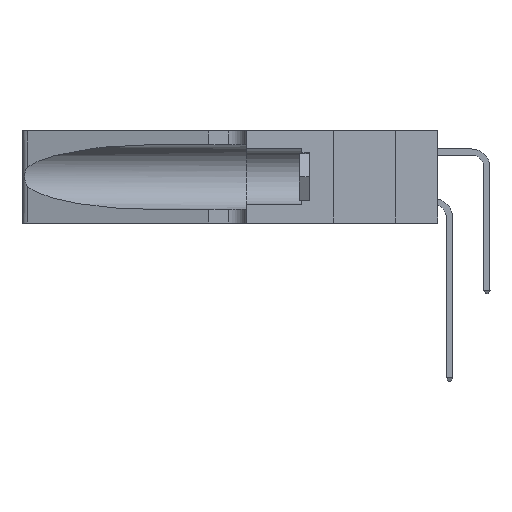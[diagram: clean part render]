
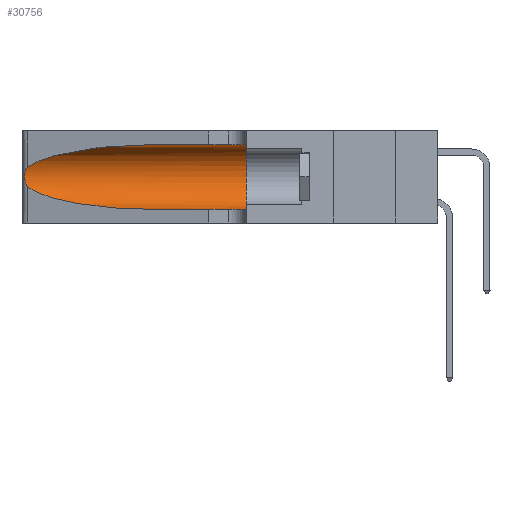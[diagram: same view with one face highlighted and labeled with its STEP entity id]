
A CAD part, left-side view. The second image highlights one B-rep face of the part: STEP entity #30756.
In plain terms, the highlighted cylindrical face has radius 3.308 mm (diameter 6.617 mm), a partial arc.
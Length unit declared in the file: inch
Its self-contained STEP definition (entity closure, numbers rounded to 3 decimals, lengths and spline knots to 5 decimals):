
#200 = ORIENTED_EDGE ( 'NONE', *, *, #23039, .F. ) ;
#329 = EDGE_CURVE ( 'NONE', #10578, #28853, #20064, .T. ) ;
#1291 = VERTEX_POINT ( 'NONE', #31344 ) ;
#1742 = CARTESIAN_POINT ( 'NONE',  ( 0.1305, 1.61858, 0.31525 ) ) ;
#2919 = CARTESIAN_POINT ( 'NONE',  ( 0.25487, 1.22718, 0.14631 ) ) ;
#3020 =( BOUNDED_CURVE ( )  B_SPLINE_CURVE ( 3, ( #16386, #25970, #28848, #18546 ),
 .UNSPECIFIED., .F., .F. ) 
 B_SPLINE_CURVE_WITH_KNOTS ( ( 4, 4 ),
 ( 3.44316, 4.71239 ),
 .UNSPECIFIED. ) 
 CURVE ( )  GEOMETRIC_REPRESENTATION_ITEM ( )  RATIONAL_B_SPLINE_CURVE ( ( 1., 0.87, 0.87, 1. ) ) 
 REPRESENTATION_ITEM ( '' )  );
#3186 = VECTOR ( 'NONE', #26799, 39.37008 ) ;
#3978 = CARTESIAN_POINT ( 'NONE',  ( 0.26075, 1.23896, 0.178 ) ) ;
#4085 = FACE_OUTER_BOUND ( 'NONE', #10664, .T. ) ;
#4154 = CARTESIAN_POINT ( 'NONE',  ( 0.1305, 1.61858, 0.05475 ) ) ;
#4290 = CARTESIAN_POINT ( 'NONE',  ( 0.25856, 1.23593, 0.16098 ) ) ;
#6045 = B_SPLINE_CURVE_WITH_KNOTS ( 'NONE', 3,
 ( #20138, #7341, #22749, #27912, #23947, #14500, #19192, #3978, #21580, #4290, #29254, #16895, #21884, #31747 ),
 .UNSPECIFIED., .F., .F.,
 ( 4, 2, 2, 2, 2, 2, 4 ),
 ( 0., 0.00027, 0.00053, 0.00107, 0.0016, 0.00187, 0.00214 ),
 .UNSPECIFIED. ) ;
#6384 = LINE ( 'NONE', #1742, #23951 ) ;
#7186 = CARTESIAN_POINT ( 'NONE',  ( 0.1305, 0.72297, 0.05475 ) ) ;
#7341 = CARTESIAN_POINT ( 'NONE',  ( 0.25555, 1.22994, 0.2215 ) ) ;
#7577 = CARTESIAN_POINT ( 'NONE',  ( 0.25487, 1.22718, 0.22369 ) ) ;
#7860 = VERTEX_POINT ( 'NONE', #31389 ) ;
#9042 = DIRECTION ( 'NONE',  ( 0., -1., 0. ) ) ;
#10578 = VERTEX_POINT ( 'NONE', #29372 ) ;
#10664 = EDGE_LOOP ( 'NONE', ( #11529, #22156, #10786, #26436, #29681, #200 ) ) ;
#10786 = ORIENTED_EDGE ( 'NONE', *, *, #19401, .T. ) ;
#11529 = ORIENTED_EDGE ( 'NONE', *, *, #329, .T. ) ;
#12019 = VERTEX_POINT ( 'NONE', #7186 ) ;
#14309 = CARTESIAN_POINT ( 'NONE',  ( 0.1305, 0.72297, 0.31525 ) ) ;
#14437 = DIRECTION ( 'NONE',  ( 0., 0., 1. ) ) ;
#14500 = CARTESIAN_POINT ( 'NONE',  ( 0.26018, 1.23835, 0.19895 ) ) ;
#14521 = CARTESIAN_POINT ( 'NONE',  ( 0.2373, 1.15595, 0.28018 ) ) ;
#15045 = AXIS2_PLACEMENT_3D ( 'NONE', #31959, #9042, #16802 ) ;
#15757 = VERTEX_POINT ( 'NONE', #2919 ) ;
#16386 = CARTESIAN_POINT ( 'NONE',  ( 0.25487, 1.22718, 0.14631 ) ) ;
#16527 = LINE ( 'NONE', #4154, #3186 ) ;
#16802 = DIRECTION ( 'NONE',  ( 0., 0., -1. ) ) ;
#16895 = CARTESIAN_POINT ( 'NONE',  ( 0.25639, 1.23186, 0.15144 ) ) ;
#17813 = EDGE_CURVE ( 'NONE', #12019, #1291, #16527, .T. ) ;
#18546 = CARTESIAN_POINT ( 'NONE',  ( 0.1305, 0.72297, 0.05475 ) ) ;
#19192 = CARTESIAN_POINT ( 'NONE',  ( 0.26075, 1.23896, 0.19203 ) ) ;
#19401 = EDGE_CURVE ( 'NONE', #15757, #12019, #3020, .T. ) ;
#20064 =( BOUNDED_CURVE ( )  B_SPLINE_CURVE ( 3, ( #14309, #21905, #14521, #7577 ),
 .UNSPECIFIED., .F., .T. ) 
 B_SPLINE_CURVE_WITH_KNOTS ( ( 4, 4 ),
 ( 1.5708, 2.84003 ),
 .UNSPECIFIED. ) 
 CURVE ( )  GEOMETRIC_REPRESENTATION_ITEM ( )  RATIONAL_B_SPLINE_CURVE ( ( 1., 0.87, 0.87, 1. ) ) 
 REPRESENTATION_ITEM ( '' )  );
#20138 = CARTESIAN_POINT ( 'NONE',  ( 0.25487, 1.22718, 0.22369 ) ) ;
#20812 = AXIS2_PLACEMENT_3D ( 'NONE', #31043, #26340, #14437 ) ;
#21580 = CARTESIAN_POINT ( 'NONE',  ( 0.26017, 1.23833, 0.17102 ) ) ;
#21596 = CIRCLE ( 'NONE', #20812, 0.13025 ) ;
#21884 = CARTESIAN_POINT ( 'NONE',  ( 0.25555, 1.22993, 0.14849 ) ) ;
#21905 = CARTESIAN_POINT ( 'NONE',  ( 0.18966, 0.96281, 0.31525 ) ) ;
#22156 = ORIENTED_EDGE ( 'NONE', *, *, #28397, .T. ) ;
#22749 = CARTESIAN_POINT ( 'NONE',  ( 0.25639, 1.23184, 0.21858 ) ) ;
#23039 = EDGE_CURVE ( 'NONE', #10578, #7860, #6384, .T. ) ;
#23947 = CARTESIAN_POINT ( 'NONE',  ( 0.25854, 1.2359, 0.20912 ) ) ;
#23951 = VECTOR ( 'NONE', #29586, 39.37008 ) ;
#23975 = CARTESIAN_POINT ( 'NONE',  ( 0.25487, 1.22718, 0.22369 ) ) ;
#25970 = CARTESIAN_POINT ( 'NONE',  ( 0.2373, 1.15595, 0.08982 ) ) ;
#26340 = DIRECTION ( 'NONE',  ( 0., 1., 0. ) ) ;
#26436 = ORIENTED_EDGE ( 'NONE', *, *, #17813, .T. ) ;
#26607 = EDGE_CURVE ( 'NONE', #7860, #1291, #21596, .T. ) ;
#26799 = DIRECTION ( 'NONE',  ( 0., -1., 0. ) ) ;
#27912 = CARTESIAN_POINT ( 'NONE',  ( 0.25787, 1.23484, 0.2124 ) ) ;
#28397 = EDGE_CURVE ( 'NONE', #28853, #15757, #6045, .T. ) ;
#28848 = CARTESIAN_POINT ( 'NONE',  ( 0.18966, 0.96281, 0.05475 ) ) ;
#28853 = VERTEX_POINT ( 'NONE', #23975 ) ;
#29155 = CYLINDRICAL_SURFACE ( 'NONE', #15045, 0.13025 ) ;
#29254 = CARTESIAN_POINT ( 'NONE',  ( 0.25789, 1.23486, 0.15765 ) ) ;
#29372 = CARTESIAN_POINT ( 'NONE',  ( 0.1305, 0.72297, 0.31525 ) ) ;
#29586 = DIRECTION ( 'NONE',  ( 0., -1., 0. ) ) ;
#29681 = ORIENTED_EDGE ( 'NONE', *, *, #26607, .F. ) ;
#30756 = ADVANCED_FACE ( 'NONE', ( #4085 ), #29155, .F. ) ;
#31043 = CARTESIAN_POINT ( 'NONE',  ( 0.1305, 0.35, 0.185 ) ) ;
#31344 = CARTESIAN_POINT ( 'NONE',  ( 0.1305, 0.35, 0.05475 ) ) ;
#31389 = CARTESIAN_POINT ( 'NONE',  ( 0.1305, 0.35, 0.31525 ) ) ;
#31747 = CARTESIAN_POINT ( 'NONE',  ( 0.25487, 1.22718, 0.14631 ) ) ;
#31959 = CARTESIAN_POINT ( 'NONE',  ( 0.1305, 1.61858, 0.185 ) ) ;
